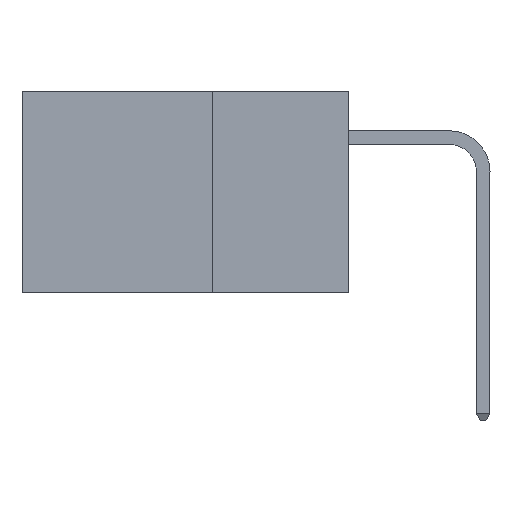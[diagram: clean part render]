
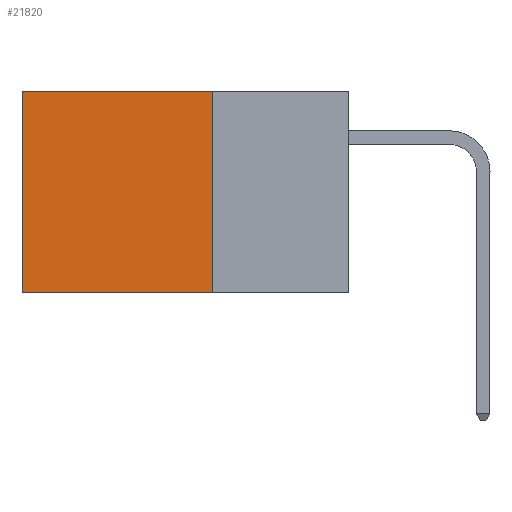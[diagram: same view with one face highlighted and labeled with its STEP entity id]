
A CAD part, left-side view. The second image highlights one B-rep face of the part: STEP entity #21820.
In plain terms, the highlighted planar face has unit normal (-1, 0, 0).
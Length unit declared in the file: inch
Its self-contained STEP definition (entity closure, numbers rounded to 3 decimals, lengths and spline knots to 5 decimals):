
#436 = VECTOR ( 'NONE', #12534, 39.37008 ) ;
#571 = DIRECTION ( 'NONE',  ( 1., 0., 0. ) ) ;
#579 = CARTESIAN_POINT ( 'NONE',  ( 0.2875, 0.6, 0. ) ) ;
#1907 = EDGE_CURVE ( 'NONE', #29551, #4039, #29296, .T. ) ;
#3417 = DIRECTION ( 'NONE',  ( 0., 1., 0. ) ) ;
#4039 = VERTEX_POINT ( 'NONE', #579 ) ;
#6200 = LINE ( 'NONE', #28509, #436 ) ;
#6998 = VECTOR ( 'NONE', #3417, 39.37008 ) ;
#9141 = EDGE_CURVE ( 'NONE', #28710, #13229, #6200, .T. ) ;
#9582 = EDGE_CURVE ( 'NONE', #29551, #28710, #22747, .T. ) ;
#12205 = CARTESIAN_POINT ( 'NONE',  ( 0.2875, 0.6, -0.37 ) ) ;
#12534 = DIRECTION ( 'NONE',  ( 0., 1., 0. ) ) ;
#13229 = VERTEX_POINT ( 'NONE', #12205 ) ;
#14432 = FACE_OUTER_BOUND ( 'NONE', #18782, .T. ) ;
#15421 = ORIENTED_EDGE ( 'NONE', *, *, #9141, .F. ) ;
#15513 = ORIENTED_EDGE ( 'NONE', *, *, #22999, .T. ) ;
#17276 = DIRECTION ( 'NONE',  ( 0., 0., -1. ) ) ;
#17434 = DIRECTION ( 'NONE',  ( 0., 0., -1. ) ) ;
#18580 = CARTESIAN_POINT ( 'NONE',  ( 0.2875, 0.25, 0. ) ) ;
#18782 = EDGE_LOOP ( 'NONE', ( #15513, #15421, #26657, #20955 ) ) ;
#19604 = AXIS2_PLACEMENT_3D ( 'NONE', #18580, #571, #25526 ) ;
#20955 = ORIENTED_EDGE ( 'NONE', *, *, #1907, .T. ) ;
#21650 = VECTOR ( 'NONE', #17434, 39.37008 ) ;
#21804 = CARTESIAN_POINT ( 'NONE',  ( 0.2875, 0.6, 0. ) ) ;
#21820 = ADVANCED_FACE ( 'NONE', ( #14432 ), #25736, .F. ) ;
#22337 = CARTESIAN_POINT ( 'NONE',  ( 0.2875, 0.25, 0. ) ) ;
#22747 = LINE ( 'NONE', #24173, #21650 ) ;
#22999 = EDGE_CURVE ( 'NONE', #4039, #13229, #25852, .T. ) ;
#24173 = CARTESIAN_POINT ( 'NONE',  ( 0.2875, 0.25, 0. ) ) ;
#25526 = DIRECTION ( 'NONE',  ( 0., 0., -1. ) ) ;
#25736 = PLANE ( 'NONE',  #19604 ) ;
#25852 = LINE ( 'NONE', #21804, #26898 ) ;
#26250 = CARTESIAN_POINT ( 'NONE',  ( 0.2875, 0.25, -0.37 ) ) ;
#26657 = ORIENTED_EDGE ( 'NONE', *, *, #9582, .F. ) ;
#26898 = VECTOR ( 'NONE', #17276, 39.37008 ) ;
#27974 = CARTESIAN_POINT ( 'NONE',  ( 0.2875, 0.25, 0. ) ) ;
#28509 = CARTESIAN_POINT ( 'NONE',  ( 0.2875, 0.25, -0.37 ) ) ;
#28710 = VERTEX_POINT ( 'NONE', #26250 ) ;
#29296 = LINE ( 'NONE', #27974, #6998 ) ;
#29551 = VERTEX_POINT ( 'NONE', #22337 ) ;
